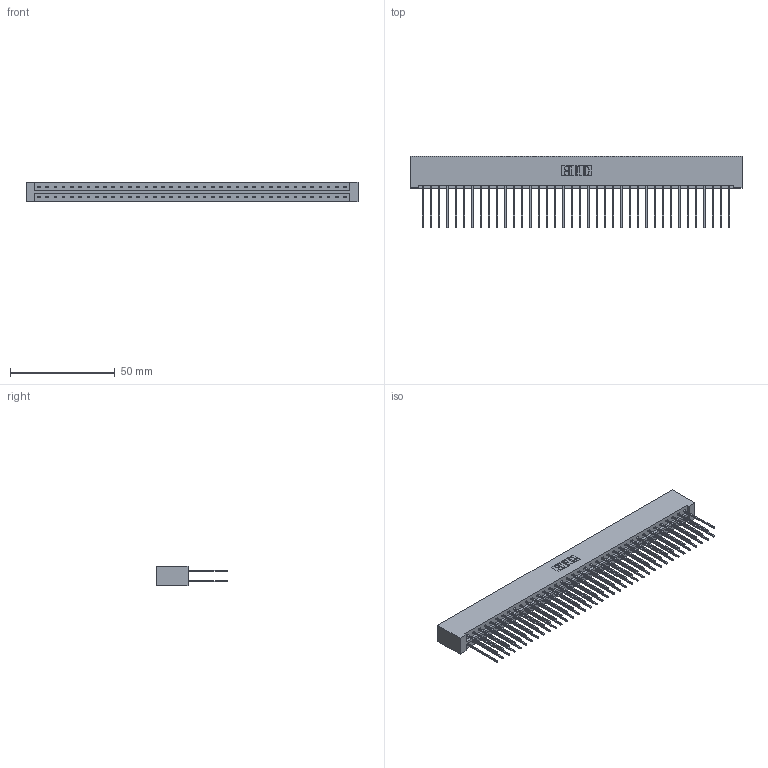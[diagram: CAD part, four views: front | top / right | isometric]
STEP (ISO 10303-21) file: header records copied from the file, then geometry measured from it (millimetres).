
FILE_DESCRIPTION (( 'STEP AP203' ), '1' );
FILE_NAME ('333-076-541-201.STEP', '2018-08-04T23:03:00', ( '' ), ( '' ), 'SwSTEP 2.0', 'SolidWorks 2016', '' );
FILE_SCHEMA (( 'CONFIG_CONTROL_DESIGN' ));
Length unit declared in the file: inch
Products named in the file (3): 333-076-541-201; 333 Part_Lugless; 345-292-001_345-293-141
Assembly tree (77 placements, depth 2):
  333-076-541-201
    333 Part_Lugless
    345-292-001_345-293-141  x76
Bounding box: 158.83 x 34.3 x 9.4 mm (x, y, z)
Volume: 17246.1 mm3; surface area: 22541.7 mm2
Topology: 77 solids, 77 shells, 4058 faces, 12067 edges, 7942 vertices
Faces by surface type: plane 2802, cylinder 1256
Entity records: 24705 total; most frequent: CARTESIAN_POINT 4098, ORIENTED_EDGE 4034, DIRECTION 3501, EDGE_CURVE 2017, VECTOR 1897, LINE 1897, VERTEX_POINT 1342, AXIS2_PLACEMENT_3D 802
